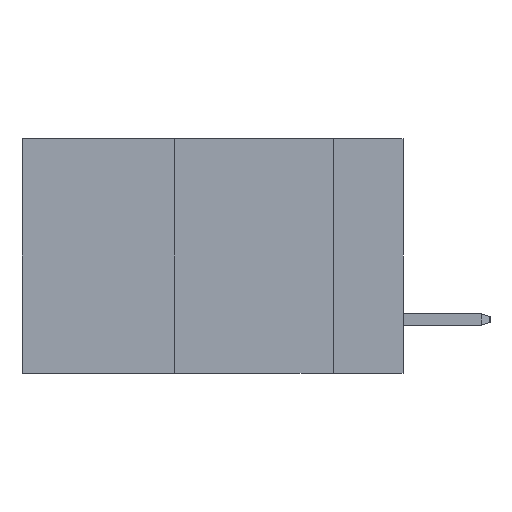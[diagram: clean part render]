
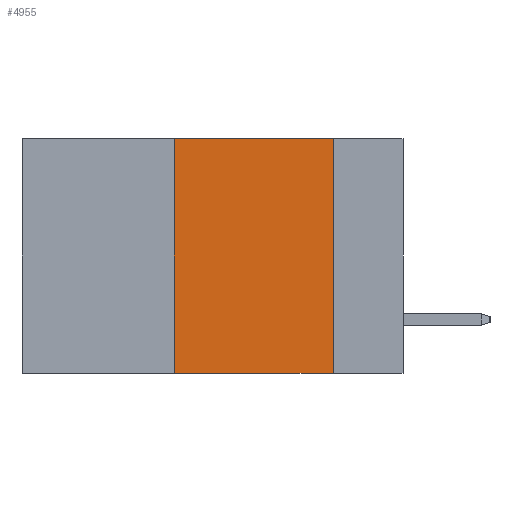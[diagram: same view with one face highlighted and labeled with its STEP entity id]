
A CAD part, left-side view. The second image highlights one B-rep face of the part: STEP entity #4955.
In plain terms, the highlighted planar face has unit normal (-1, 0, 0).
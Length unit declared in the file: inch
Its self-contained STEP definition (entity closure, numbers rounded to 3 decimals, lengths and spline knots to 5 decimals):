
#275 = CARTESIAN_POINT ( 'NONE',  ( 0., 0.36, 0. ) ) ;
#364 = CARTESIAN_POINT ( 'NONE',  ( 0., 0.36, -0.37 ) ) ;
#415 = CARTESIAN_POINT ( 'NONE',  ( 0., 0.6, 0. ) ) ;
#431 = ORIENTED_EDGE ( 'NONE', *, *, #5576, .T. ) ;
#1619 = DIRECTION ( 'NONE',  ( 0., -1., 0. ) ) ;
#1873 = DIRECTION ( 'NONE',  ( 0., 0., 1. ) ) ;
#1961 = DIRECTION ( 'NONE',  ( 1., 0., 0. ) ) ;
#2426 = CARTESIAN_POINT ( 'NONE',  ( 0., 0.6, 0. ) ) ;
#2510 = VECTOR ( 'NONE', #9878, 39.37008 ) ;
#2604 = ORIENTED_EDGE ( 'NONE', *, *, #3306, .F. ) ;
#2769 = PLANE ( 'NONE',  #5457 ) ;
#2873 = FACE_OUTER_BOUND ( 'NONE', #9085, .T. ) ;
#3306 = EDGE_CURVE ( 'NONE', #8414, #5368, #7288, .T. ) ;
#3598 = CARTESIAN_POINT ( 'NONE',  ( 0., 0.11, -0.37 ) ) ;
#4311 = CARTESIAN_POINT ( 'NONE',  ( 0., 0.11, 0. ) ) ;
#4425 = CARTESIAN_POINT ( 'NONE',  ( 0., 0.6, -0.37 ) ) ;
#4427 = ORIENTED_EDGE ( 'NONE', *, *, #8209, .F. ) ;
#4430 = VECTOR ( 'NONE', #1873, 39.37008 ) ;
#4922 = EDGE_CURVE ( 'NONE', #5727, #8619, #9031, .T. ) ;
#4955 = ADVANCED_FACE ( 'NONE', ( #2873 ), #2769, .F. ) ;
#5132 = DIRECTION ( 'NONE',  ( 0., 0., -1. ) ) ;
#5368 = VERTEX_POINT ( 'NONE', #9265 ) ;
#5457 = AXIS2_PLACEMENT_3D ( 'NONE', #415, #1961, #5132 ) ;
#5576 = EDGE_CURVE ( 'NONE', #8414, #8619, #9838, .T. ) ;
#5727 = VERTEX_POINT ( 'NONE', #10135 ) ;
#7288 = LINE ( 'NONE', #275, #4430 ) ;
#8155 = ORIENTED_EDGE ( 'NONE', *, *, #4922, .F. ) ;
#8209 = EDGE_CURVE ( 'NONE', #5368, #5727, #10139, .T. ) ;
#8414 = VERTEX_POINT ( 'NONE', #364 ) ;
#8619 = VERTEX_POINT ( 'NONE', #3598 ) ;
#9031 = LINE ( 'NONE', #4311, #2510 ) ;
#9085 = EDGE_LOOP ( 'NONE', ( #8155, #4427, #2604, #431 ) ) ;
#9193 = DIRECTION ( 'NONE',  ( 0., -1., 0. ) ) ;
#9265 = CARTESIAN_POINT ( 'NONE',  ( 0., 0.36, 0. ) ) ;
#9401 = VECTOR ( 'NONE', #9193, 39.37008 ) ;
#9774 = VECTOR ( 'NONE', #1619, 39.37008 ) ;
#9838 = LINE ( 'NONE', #4425, #9401 ) ;
#9878 = DIRECTION ( 'NONE',  ( 0., 0., -1. ) ) ;
#10135 = CARTESIAN_POINT ( 'NONE',  ( 0., 0.11, 0. ) ) ;
#10139 = LINE ( 'NONE', #2426, #9774 ) ;
